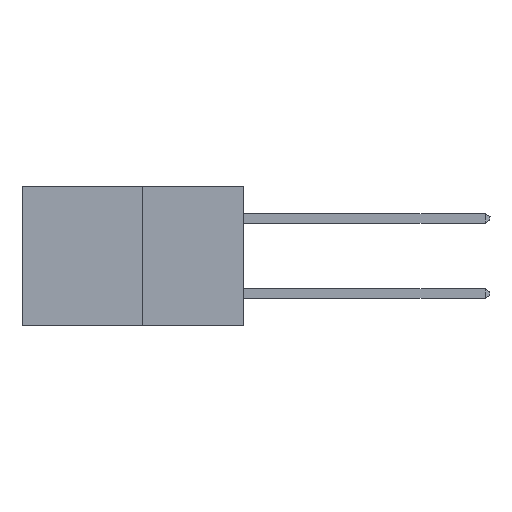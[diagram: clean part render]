
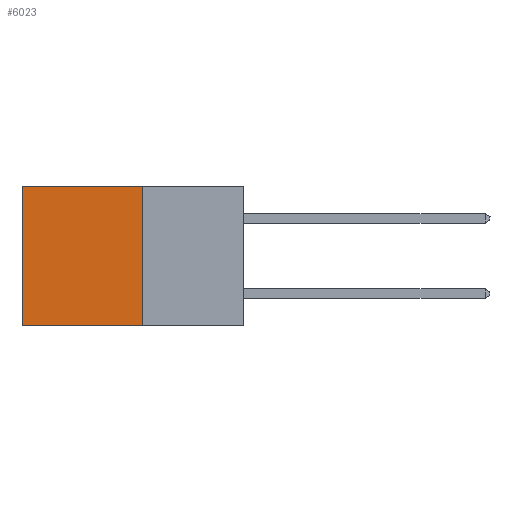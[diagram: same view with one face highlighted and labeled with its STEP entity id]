
A CAD part, left-side view. The second image highlights one B-rep face of the part: STEP entity #6023.
In plain terms, the highlighted planar face has unit normal (-1, 0, 0).
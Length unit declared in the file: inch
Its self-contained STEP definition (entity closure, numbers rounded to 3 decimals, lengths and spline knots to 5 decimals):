
#234 = LINE ( 'NONE', #10617, #17913 ) ;
#470 = CARTESIAN_POINT ( 'NONE',  ( 0.277, 0.59, 0. ) ) ;
#3264 = ORIENTED_EDGE ( 'NONE', *, *, #6652, .F. ) ;
#4503 = VECTOR ( 'NONE', #11356, 39.37008 ) ;
#4539 = EDGE_CURVE ( 'NONE', #24675, #15337, #20800, .T. ) ;
#5508 = EDGE_CURVE ( 'NONE', #15337, #24537, #234, .T. ) ;
#6023 = ADVANCED_FACE ( 'NONE', ( #10357 ), #23524, .F. ) ;
#6652 = EDGE_CURVE ( 'NONE', #19867, #24537, #10674, .T. ) ;
#6929 = DIRECTION ( 'NONE',  ( 0., 0., -1. ) ) ;
#7782 = CARTESIAN_POINT ( 'NONE',  ( 0.277, 0.27, -0.37 ) ) ;
#7894 = AXIS2_PLACEMENT_3D ( 'NONE', #23427, #23031, #22732 ) ;
#8801 = CARTESIAN_POINT ( 'NONE',  ( 0.277, 0.59, -0.37 ) ) ;
#9540 = VECTOR ( 'NONE', #28315, 39.37008 ) ;
#10357 = FACE_OUTER_BOUND ( 'NONE', #26568, .T. ) ;
#10535 = CARTESIAN_POINT ( 'NONE',  ( 0.277, 0.27, -0.37 ) ) ;
#10617 = CARTESIAN_POINT ( 'NONE',  ( 0.277, 0.59, -0.37 ) ) ;
#10674 = LINE ( 'NONE', #10535, #4503 ) ;
#10839 = ORIENTED_EDGE ( 'NONE', *, *, #24233, .F. ) ;
#11356 = DIRECTION ( 'NONE',  ( 0., 1., 0. ) ) ;
#11717 = LINE ( 'NONE', #14653, #9540 ) ;
#14653 = CARTESIAN_POINT ( 'NONE',  ( 0.277, 0.27, -0.37 ) ) ;
#14734 = VECTOR ( 'NONE', #24608, 39.37008 ) ;
#15337 = VERTEX_POINT ( 'NONE', #470 ) ;
#17913 = VECTOR ( 'NONE', #6929, 39.37008 ) ;
#18343 = CARTESIAN_POINT ( 'NONE',  ( 0.277, 0.27, 0. ) ) ;
#19867 = VERTEX_POINT ( 'NONE', #7782 ) ;
#20800 = LINE ( 'NONE', #23804, #14734 ) ;
#22732 = DIRECTION ( 'NONE',  ( 0., 0., -1. ) ) ;
#23031 = DIRECTION ( 'NONE',  ( 1., 0., 0. ) ) ;
#23427 = CARTESIAN_POINT ( 'NONE',  ( 0.277, 0.27, -0.37 ) ) ;
#23524 = PLANE ( 'NONE',  #7894 ) ;
#23804 = CARTESIAN_POINT ( 'NONE',  ( 0.277, 0.27, 0. ) ) ;
#24233 = EDGE_CURVE ( 'NONE', #24675, #19867, #11717, .T. ) ;
#24537 = VERTEX_POINT ( 'NONE', #8801 ) ;
#24608 = DIRECTION ( 'NONE',  ( 0., 1., 0. ) ) ;
#24675 = VERTEX_POINT ( 'NONE', #18343 ) ;
#25188 = ORIENTED_EDGE ( 'NONE', *, *, #5508, .T. ) ;
#25623 = ORIENTED_EDGE ( 'NONE', *, *, #4539, .T. ) ;
#26568 = EDGE_LOOP ( 'NONE', ( #25188, #3264, #10839, #25623 ) ) ;
#28315 = DIRECTION ( 'NONE',  ( 0., 0., -1. ) ) ;
